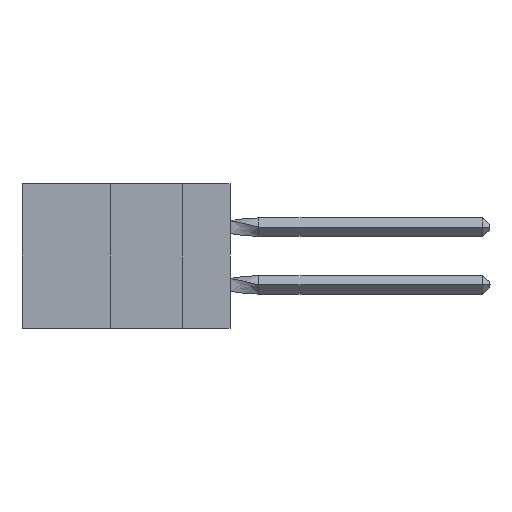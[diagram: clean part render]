
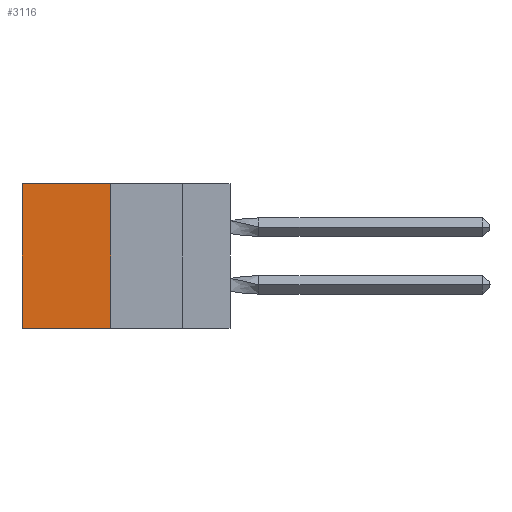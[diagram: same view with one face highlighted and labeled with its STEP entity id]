
A CAD part, left-side view. The second image highlights one B-rep face of the part: STEP entity #3116.
In plain terms, the highlighted planar face has unit normal (-1, 0, 0).
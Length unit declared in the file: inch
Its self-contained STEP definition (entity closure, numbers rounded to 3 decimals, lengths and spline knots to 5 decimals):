
#476 = PLANE ( 'NONE',  #10372 ) ;
#519 = EDGE_LOOP ( 'NONE', ( #12609, #14012, #12013, #13419 ) ) ;
#1507 = CARTESIAN_POINT ( 'NONE',  ( 0.305, 0.413, -0.5 ) ) ;
#1996 = LINE ( 'NONE', #15631, #15976 ) ;
#2451 = DIRECTION ( 'NONE',  ( 0., 0., -1. ) ) ;
#2891 = LINE ( 'NONE', #15883, #3690 ) ;
#3116 = ADVANCED_FACE ( 'NONE', ( #11159 ), #476, .F. ) ;
#3690 = VECTOR ( 'NONE', #7042, 39.37008 ) ;
#3850 = VECTOR ( 'NONE', #12983, 39.37008 ) ;
#5405 = EDGE_CURVE ( 'NONE', #11074, #5589, #1996, .T. ) ;
#5589 = VERTEX_POINT ( 'NONE', #10672 ) ;
#6742 = DIRECTION ( 'NONE',  ( 0., 0., -1. ) ) ;
#7042 = DIRECTION ( 'NONE',  ( 0., 1., 0. ) ) ;
#7213 = LINE ( 'NONE', #10385, #3850 ) ;
#7921 = DIRECTION ( 'NONE',  ( 1., 0., 0. ) ) ;
#9112 = CARTESIAN_POINT ( 'NONE',  ( 0.305, 0.72, 0. ) ) ;
#9226 = LINE ( 'NONE', #9969, #12596 ) ;
#9871 = EDGE_CURVE ( 'NONE', #10468, #14824, #9226, .T. ) ;
#9969 = CARTESIAN_POINT ( 'NONE',  ( 0.305, 0.413, -0.5 ) ) ;
#10082 = CARTESIAN_POINT ( 'NONE',  ( 0.305, 0.413, 0. ) ) ;
#10372 = AXIS2_PLACEMENT_3D ( 'NONE', #14305, #7921, #13050 ) ;
#10385 = CARTESIAN_POINT ( 'NONE',  ( 0.305, 0.413, 0. ) ) ;
#10468 = VERTEX_POINT ( 'NONE', #10082 ) ;
#10672 = CARTESIAN_POINT ( 'NONE',  ( 0.305, 0.72, -0.5 ) ) ;
#11074 = VERTEX_POINT ( 'NONE', #9112 ) ;
#11159 = FACE_OUTER_BOUND ( 'NONE', #519, .T. ) ;
#11466 = EDGE_CURVE ( 'NONE', #14824, #5589, #2891, .T. ) ;
#12013 = ORIENTED_EDGE ( 'NONE', *, *, #9871, .F. ) ;
#12596 = VECTOR ( 'NONE', #2451, 39.37008 ) ;
#12609 = ORIENTED_EDGE ( 'NONE', *, *, #5405, .T. ) ;
#12983 = DIRECTION ( 'NONE',  ( 0., 1., 0. ) ) ;
#13050 = DIRECTION ( 'NONE',  ( 0., 0., -1. ) ) ;
#13419 = ORIENTED_EDGE ( 'NONE', *, *, #14834, .T. ) ;
#14012 = ORIENTED_EDGE ( 'NONE', *, *, #11466, .F. ) ;
#14305 = CARTESIAN_POINT ( 'NONE',  ( 0.305, 0.413, -0.5 ) ) ;
#14824 = VERTEX_POINT ( 'NONE', #1507 ) ;
#14834 = EDGE_CURVE ( 'NONE', #10468, #11074, #7213, .T. ) ;
#15631 = CARTESIAN_POINT ( 'NONE',  ( 0.305, 0.72, -0.5 ) ) ;
#15883 = CARTESIAN_POINT ( 'NONE',  ( 0.305, 0.413, -0.5 ) ) ;
#15976 = VECTOR ( 'NONE', #6742, 39.37008 ) ;
